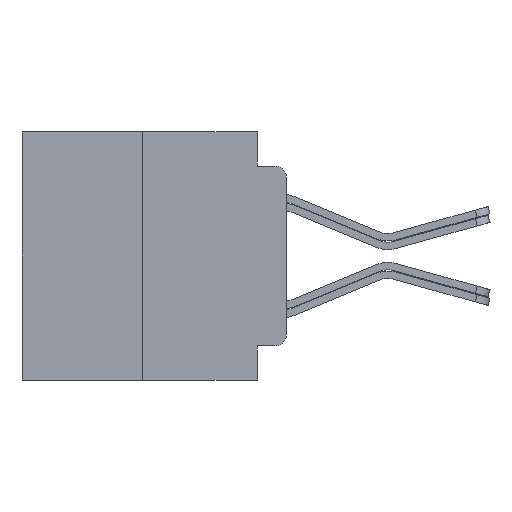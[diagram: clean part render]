
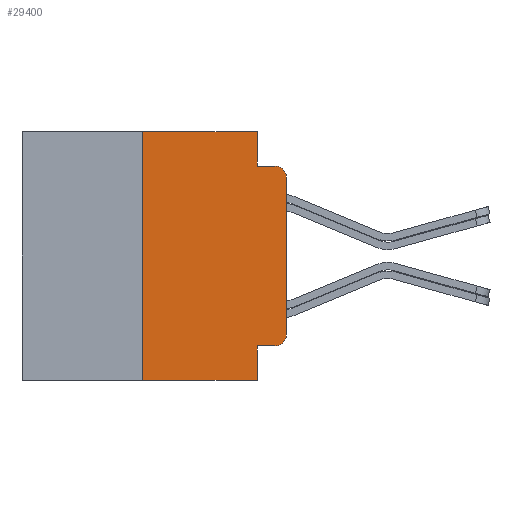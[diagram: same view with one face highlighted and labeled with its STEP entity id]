
A CAD part, left-side view. The second image highlights one B-rep face of the part: STEP entity #29400.
In plain terms, the highlighted planar face has unit normal (-1, 0, 0).
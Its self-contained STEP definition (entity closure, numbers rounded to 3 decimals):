
#51 = EDGE_CURVE ( 'NONE', #16103, #15428, #3063, .T. ) ;
#1294 = DIRECTION ( 'NONE',  ( 0., 0., 1. ) ) ;
#1933 = DIRECTION ( 'NONE',  ( 0., 0., -1. ) ) ;
#2121 = CARTESIAN_POINT ( 'NONE',  ( -75.603, 0.508, -3.975 ) ) ;
#2310 = LINE ( 'NONE', #26855, #26142 ) ;
#2696 = VERTEX_POINT ( 'NONE', #3277 ) ;
#3063 = LINE ( 'NONE', #4554, #9903 ) ;
#3277 = CARTESIAN_POINT ( 'NONE',  ( -75.603, 6.35, -5.486 ) ) ;
#4030 = CARTESIAN_POINT ( 'NONE',  ( -75.603, 1.295, 3.975 ) ) ;
#4073 = LINE ( 'NONE', #17567, #21739 ) ;
#4533 = AXIS2_PLACEMENT_3D ( 'NONE', #13018, #13115, #11081 ) ;
#4554 = CARTESIAN_POINT ( 'NONE',  ( -75.603, 1.295, 3.975 ) ) ;
#4668 = CARTESIAN_POINT ( 'NONE',  ( -75.603, 1.295, -3.975 ) ) ;
#4780 = VERTEX_POINT ( 'NONE', #22982 ) ;
#5117 = CARTESIAN_POINT ( 'NONE',  ( -75.603, 0.508, -3.467 ) ) ;
#5203 = DIRECTION ( 'NONE',  ( 0., 0., -1. ) ) ;
#5754 = LINE ( 'NONE', #27683, #22009 ) ;
#5840 = DIRECTION ( 'NONE',  ( 0., -1., 0. ) ) ;
#6141 = CARTESIAN_POINT ( 'NONE',  ( -75.603, 0., 5.486 ) ) ;
#6191 = EDGE_CURVE ( 'NONE', #9021, #17872, #15047, .T. ) ;
#6372 = ORIENTED_EDGE ( 'NONE', *, *, #6191, .F. ) ;
#6512 = CARTESIAN_POINT ( 'NONE',  ( -75.603, 1.295, -3.975 ) ) ;
#6606 = AXIS2_PLACEMENT_3D ( 'NONE', #16941, #12085, #5203 ) ;
#6931 = ORIENTED_EDGE ( 'NONE', *, *, #12163, .F. ) ;
#8321 = ORIENTED_EDGE ( 'NONE', *, *, #28411, .F. ) ;
#8452 = ORIENTED_EDGE ( 'NONE', *, *, #23914, .F. ) ;
#9021 = VERTEX_POINT ( 'NONE', #27527 ) ;
#9903 = VECTOR ( 'NONE', #25454, 1000. ) ;
#9922 = EDGE_CURVE ( 'NONE', #4780, #15428, #22902, .T. ) ;
#10620 = VERTEX_POINT ( 'NONE', #2121 ) ;
#11081 = DIRECTION ( 'NONE',  ( 0., 0., -1. ) ) ;
#11352 = DIRECTION ( 'NONE',  ( 0., -1., 0. ) ) ;
#11651 = EDGE_CURVE ( 'NONE', #10620, #25100, #18522, .T. ) ;
#11654 = DIRECTION ( 'NONE',  ( 0., 0., -1. ) ) ;
#11835 = FACE_OUTER_BOUND ( 'NONE', #28856, .T. ) ;
#11995 = ORIENTED_EDGE ( 'NONE', *, *, #26986, .T. ) ;
#12085 = DIRECTION ( 'NONE',  ( -1., 0., 0. ) ) ;
#12163 = EDGE_CURVE ( 'NONE', #2696, #9021, #18125, .T. ) ;
#12995 = EDGE_CURVE ( 'NONE', #25100, #4780, #28160, .T. ) ;
#13018 = CARTESIAN_POINT ( 'NONE',  ( -75.603, 11.684, 5.486 ) ) ;
#13115 = DIRECTION ( 'NONE',  ( 1., 0., 0. ) ) ;
#13881 = VERTEX_POINT ( 'NONE', #4668 ) ;
#14346 = ORIENTED_EDGE ( 'NONE', *, *, #51, .F. ) ;
#14539 = CARTESIAN_POINT ( 'NONE',  ( -75.603, 1.295, -5.486 ) ) ;
#14969 = AXIS2_PLACEMENT_3D ( 'NONE', #5117, #16352, #24512 ) ;
#15002 = CARTESIAN_POINT ( 'NONE',  ( -75.603, 0., -3.467 ) ) ;
#15047 = LINE ( 'NONE', #26874, #20454 ) ;
#15090 = DIRECTION ( 'NONE',  ( 0., -1., 0. ) ) ;
#15428 = VERTEX_POINT ( 'NONE', #24074 ) ;
#15619 = EDGE_CURVE ( 'NONE', #13881, #10620, #25597, .T. ) ;
#15900 = VERTEX_POINT ( 'NONE', #14539 ) ;
#16103 = VERTEX_POINT ( 'NONE', #4030 ) ;
#16352 = DIRECTION ( 'NONE',  ( -1., 0., 0. ) ) ;
#16941 = CARTESIAN_POINT ( 'NONE',  ( -75.603, 0.508, 3.467 ) ) ;
#17567 = CARTESIAN_POINT ( 'NONE',  ( -75.603, 11.684, -5.486 ) ) ;
#17769 = PLANE ( 'NONE',  #4533 ) ;
#17872 = VERTEX_POINT ( 'NONE', #29269 ) ;
#18125 = LINE ( 'NONE', #27593, #27844 ) ;
#18522 = CIRCLE ( 'NONE', #14969, 0.508 ) ;
#18693 = ORIENTED_EDGE ( 'NONE', *, *, #15619, .T. ) ;
#19844 = VECTOR ( 'NONE', #11352, 1000. ) ;
#20454 = VECTOR ( 'NONE', #15090, 1000. ) ;
#20568 = DIRECTION ( 'NONE',  ( 0., 0., 1. ) ) ;
#21739 = VECTOR ( 'NONE', #5840, 1000. ) ;
#22009 = VECTOR ( 'NONE', #11654, 1000. ) ;
#22046 = VECTOR ( 'NONE', #1294, 1000. ) ;
#22902 = CIRCLE ( 'NONE', #6606, 0.508 ) ;
#22973 = ORIENTED_EDGE ( 'NONE', *, *, #9922, .T. ) ;
#22982 = CARTESIAN_POINT ( 'NONE',  ( -75.603, 0., 3.467 ) ) ;
#23277 = ORIENTED_EDGE ( 'NONE', *, *, #11651, .T. ) ;
#23904 = ORIENTED_EDGE ( 'NONE', *, *, #12995, .T. ) ;
#23914 = EDGE_CURVE ( 'NONE', #13881, #15900, #2310, .T. ) ;
#24074 = CARTESIAN_POINT ( 'NONE',  ( -75.603, 0.508, 3.975 ) ) ;
#24512 = DIRECTION ( 'NONE',  ( 0., 0., -1. ) ) ;
#25100 = VERTEX_POINT ( 'NONE', #15002 ) ;
#25454 = DIRECTION ( 'NONE',  ( 0., -1., 0. ) ) ;
#25597 = LINE ( 'NONE', #6512, #19844 ) ;
#26142 = VECTOR ( 'NONE', #1933, 1000. ) ;
#26855 = CARTESIAN_POINT ( 'NONE',  ( -75.603, 1.295, 0. ) ) ;
#26874 = CARTESIAN_POINT ( 'NONE',  ( -75.603, 11.684, 5.486 ) ) ;
#26986 = EDGE_CURVE ( 'NONE', #2696, #15900, #4073, .T. ) ;
#27527 = CARTESIAN_POINT ( 'NONE',  ( -75.603, 6.35, 5.486 ) ) ;
#27593 = CARTESIAN_POINT ( 'NONE',  ( -75.603, 6.35, -5.486 ) ) ;
#27683 = CARTESIAN_POINT ( 'NONE',  ( -75.603, 1.295, 0. ) ) ;
#27844 = VECTOR ( 'NONE', #20568, 1000. ) ;
#28160 = LINE ( 'NONE', #6141, #22046 ) ;
#28411 = EDGE_CURVE ( 'NONE', #17872, #16103, #5754, .T. ) ;
#28856 = EDGE_LOOP ( 'NONE', ( #18693, #23277, #23904, #22973, #14346, #8321, #6372, #6931, #11995, #8452 ) ) ;
#29269 = CARTESIAN_POINT ( 'NONE',  ( -75.603, 1.295, 5.486 ) ) ;
#29400 = ADVANCED_FACE ( 'NONE', ( #11835 ), #17769, .F. ) ;
